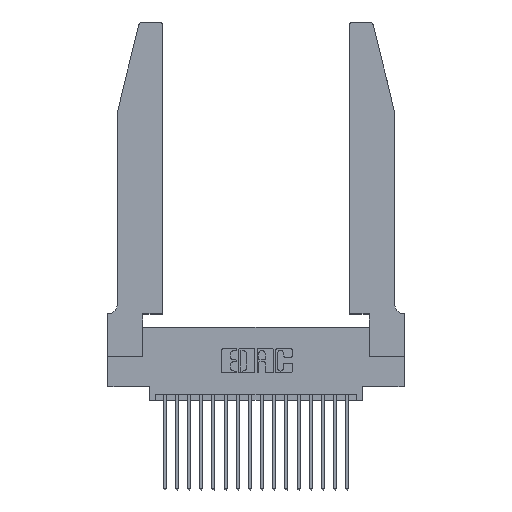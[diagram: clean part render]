
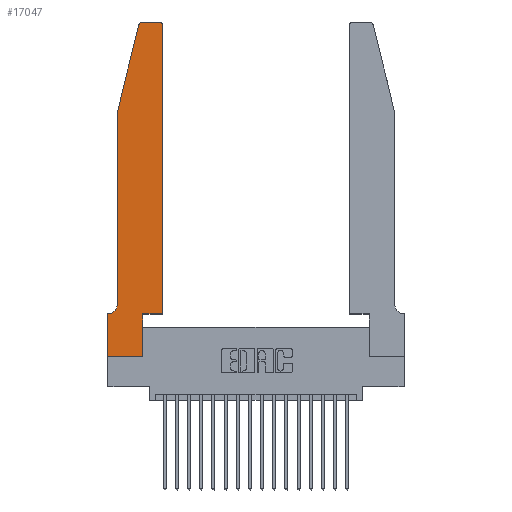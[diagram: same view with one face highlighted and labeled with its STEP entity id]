
A CAD part, top view. The second image highlights one B-rep face of the part: STEP entity #17047.
In plain terms, the highlighted planar face has unit normal (0, 0, 1).
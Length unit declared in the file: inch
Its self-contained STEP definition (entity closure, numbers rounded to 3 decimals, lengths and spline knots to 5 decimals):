
#54 = EDGE_CURVE ( 'NONE', #509, #8735, #18047, .T. ) ;
#371 = ORIENTED_EDGE ( 'NONE', *, *, #1451, .T. ) ;
#509 = VERTEX_POINT ( 'NONE', #17318 ) ;
#951 = VECTOR ( 'NONE', #1457, 39.37008 ) ;
#1002 = DIRECTION ( 'NONE',  ( 0., 0., 1. ) ) ;
#1340 = DIRECTION ( 'NONE',  ( 0., 0., 1. ) ) ;
#1374 = LINE ( 'NONE', #19418, #10058 ) ;
#1417 = VERTEX_POINT ( 'NONE', #4152 ) ;
#1451 = EDGE_CURVE ( 'NONE', #13313, #13739, #20939, .T. ) ;
#1457 = DIRECTION ( 'NONE',  ( 1., 0., 0. ) ) ;
#1460 = CARTESIAN_POINT ( 'NONE',  ( 0.2865, 0.35, 0.37 ) ) ;
#1498 = LINE ( 'NONE', #16022, #951 ) ;
#1905 = ORIENTED_EDGE ( 'NONE', *, *, #6843, .T. ) ;
#2422 = ORIENTED_EDGE ( 'NONE', *, *, #19649, .T. ) ;
#2822 = VERTEX_POINT ( 'NONE', #12686 ) ;
#2875 = VERTEX_POINT ( 'NONE', #12824 ) ;
#3305 = EDGE_CURVE ( 'NONE', #2822, #9275, #16596, .T. ) ;
#3934 = DIRECTION ( 'NONE',  ( -1., 0., 0. ) ) ;
#4152 = CARTESIAN_POINT ( 'NONE',  ( 0.4505, 2.72, 0.37 ) ) ;
#4226 = VECTOR ( 'NONE', #3934, 39.37008 ) ;
#5204 = DIRECTION ( 'NONE',  ( 0., 0., -1. ) ) ;
#5249 = EDGE_CURVE ( 'NONE', #1417, #8961, #20231, .T. ) ;
#5583 = DIRECTION ( 'NONE',  ( 1., 0., 0. ) ) ;
#5723 = DIRECTION ( 'NONE',  ( -0.239, -0.971, 0. ) ) ;
#6081 = CARTESIAN_POINT ( 'NONE',  ( 0.4205, 2.75, 0.37 ) ) ;
#6629 = DIRECTION ( 'NONE',  ( 0., 1., 0. ) ) ;
#6688 = CARTESIAN_POINT ( 'NONE',  ( 0.2865, 0.35, 0.37 ) ) ;
#6843 = EDGE_CURVE ( 'NONE', #2875, #13313, #9479, .T. ) ;
#7034 = VECTOR ( 'NONE', #5723, 39.37008 ) ;
#7166 = CARTESIAN_POINT ( 'NONE',  ( 0.2605, 2.75, 0.37 ) ) ;
#7242 = CARTESIAN_POINT ( 'NONE',  ( 0., 0., 0.37 ) ) ;
#7247 = ORIENTED_EDGE ( 'NONE', *, *, #15162, .T. ) ;
#7620 = DIRECTION ( 'NONE',  ( 0., -1., 0. ) ) ;
#7765 = CARTESIAN_POINT ( 'NONE',  ( 0.4505, 0.35, 0.37 ) ) ;
#8170 = CARTESIAN_POINT ( 'NONE',  ( 0.25487, 2.72718, 0.37 ) ) ;
#8223 = VECTOR ( 'NONE', #8374, 39.37008 ) ;
#8374 = DIRECTION ( 'NONE',  ( 0., 1., 0. ) ) ;
#8735 = VERTEX_POINT ( 'NONE', #11667 ) ;
#8888 = CARTESIAN_POINT ( 'NONE',  ( 0.284, 2.75, 0.37 ) ) ;
#8961 = VERTEX_POINT ( 'NONE', #6081 ) ;
#9033 = CARTESIAN_POINT ( 'NONE',  ( 0.0755, 0.35, 0.37 ) ) ;
#9182 = ORIENTED_EDGE ( 'NONE', *, *, #15832, .T. ) ;
#9275 = VERTEX_POINT ( 'NONE', #19882 ) ;
#9479 = LINE ( 'NONE', #7242, #17491 ) ;
#9897 = AXIS2_PLACEMENT_3D ( 'NONE', #11082, #1340, #12687 ) ;
#10058 = VECTOR ( 'NONE', #6629, 39.37008 ) ;
#10144 = EDGE_LOOP ( 'NONE', ( #12429, #12339, #7247, #16080, #9182, #13058, #18904, #1905, #371, #14079, #2422, #13237 ) ) ;
#10799 = CARTESIAN_POINT ( 'NONE',  ( 0.284, 2.72, 0.37 ) ) ;
#10804 = LINE ( 'NONE', #16924, #7034 ) ;
#11005 = CIRCLE ( 'NONE', #20315, 0.07 ) ;
#11082 = CARTESIAN_POINT ( 'NONE',  ( 0.4205, 2.72, 0.37 ) ) ;
#11240 = DIRECTION ( 'NONE',  ( 0., -1., 0. ) ) ;
#11667 = CARTESIAN_POINT ( 'NONE',  ( 0.0755, 0.42, 0.37 ) ) ;
#11940 = PLANE ( 'NONE',  #12988 ) ;
#12044 = EDGE_CURVE ( 'NONE', #14574, #12271, #12161, .T. ) ;
#12161 = CIRCLE ( 'NONE', #19361, 0.03 ) ;
#12206 = EDGE_CURVE ( 'NONE', #13739, #19024, #1498, .T. ) ;
#12271 = VERTEX_POINT ( 'NONE', #8170 ) ;
#12339 = ORIENTED_EDGE ( 'NONE', *, *, #12044, .T. ) ;
#12374 = DIRECTION ( 'NONE',  ( 1., 0., 0. ) ) ;
#12429 = ORIENTED_EDGE ( 'NONE', *, *, #15981, .T. ) ;
#12686 = CARTESIAN_POINT ( 'NONE',  ( 0.0055, 0.35, 0.37 ) ) ;
#12687 = DIRECTION ( 'NONE',  ( 1., 0., 0. ) ) ;
#12824 = CARTESIAN_POINT ( 'NONE',  ( 0., 0., 0.37 ) ) ;
#12909 = EDGE_CURVE ( 'NONE', #9275, #2875, #17894, .T. ) ;
#12988 = AXIS2_PLACEMENT_3D ( 'NONE', #13561, #15177, #5583 ) ;
#13058 = ORIENTED_EDGE ( 'NONE', *, *, #3305, .T. ) ;
#13237 = ORIENTED_EDGE ( 'NONE', *, *, #5249, .T. ) ;
#13313 = VERTEX_POINT ( 'NONE', #13633 ) ;
#13561 = CARTESIAN_POINT ( 'NONE',  ( 0., 0.35, 0.37 ) ) ;
#13633 = CARTESIAN_POINT ( 'NONE',  ( 0.2865, 0., 0.37 ) ) ;
#13639 = VECTOR ( 'NONE', #7620, 39.37008 ) ;
#13739 = VERTEX_POINT ( 'NONE', #6688 ) ;
#14079 = ORIENTED_EDGE ( 'NONE', *, *, #12206, .T. ) ;
#14391 = CARTESIAN_POINT ( 'NONE',  ( 0.0755, 2., 0.37 ) ) ;
#14574 = VERTEX_POINT ( 'NONE', #8888 ) ;
#14793 = CARTESIAN_POINT ( 'NONE',  ( 0.0055, 0.42, 0.37 ) ) ;
#14879 = FACE_OUTER_BOUND ( 'NONE', #10144, .T. ) ;
#15162 = EDGE_CURVE ( 'NONE', #12271, #509, #10804, .T. ) ;
#15177 = DIRECTION ( 'NONE',  ( 0., 0., 1. ) ) ;
#15415 = DIRECTION ( 'NONE',  ( -1., 0., 0. ) ) ;
#15611 = CARTESIAN_POINT ( 'NONE',  ( 0., 0., 0.37 ) ) ;
#15832 = EDGE_CURVE ( 'NONE', #8735, #2822, #11005, .T. ) ;
#15981 = EDGE_CURVE ( 'NONE', #8961, #14574, #20718, .T. ) ;
#16022 = CARTESIAN_POINT ( 'NONE',  ( 0.4505, 0.35, 0.37 ) ) ;
#16080 = ORIENTED_EDGE ( 'NONE', *, *, #54, .T. ) ;
#16410 = DIRECTION ( 'NONE',  ( -1., 0., 0. ) ) ;
#16596 = LINE ( 'NONE', #9033, #20311 ) ;
#16924 = CARTESIAN_POINT ( 'NONE',  ( 0.0755, 2., 0.37 ) ) ;
#17047 = ADVANCED_FACE ( 'NONE', ( #14879 ), #11940, .T. ) ;
#17318 = CARTESIAN_POINT ( 'NONE',  ( 0.0755, 2., 0.37 ) ) ;
#17491 = VECTOR ( 'NONE', #18590, 39.37008 ) ;
#17556 = VECTOR ( 'NONE', #11240, 39.37008 ) ;
#17894 = LINE ( 'NONE', #15611, #13639 ) ;
#18047 = LINE ( 'NONE', #14391, #17556 ) ;
#18590 = DIRECTION ( 'NONE',  ( 1., 0., 0. ) ) ;
#18904 = ORIENTED_EDGE ( 'NONE', *, *, #12909, .T. ) ;
#19024 = VERTEX_POINT ( 'NONE', #7765 ) ;
#19361 = AXIS2_PLACEMENT_3D ( 'NONE', #10799, #1002, #12374 ) ;
#19418 = CARTESIAN_POINT ( 'NONE',  ( 0.4505, 0.35, 0.37 ) ) ;
#19649 = EDGE_CURVE ( 'NONE', #19024, #1417, #1374, .T. ) ;
#19882 = CARTESIAN_POINT ( 'NONE',  ( 0., 0.35, 0.37 ) ) ;
#20231 = CIRCLE ( 'NONE', #9897, 0.03 ) ;
#20311 = VECTOR ( 'NONE', #15415, 39.37008 ) ;
#20315 = AXIS2_PLACEMENT_3D ( 'NONE', #14793, #5204, #16410 ) ;
#20718 = LINE ( 'NONE', #7166, #4226 ) ;
#20939 = LINE ( 'NONE', #1460, #8223 ) ;
